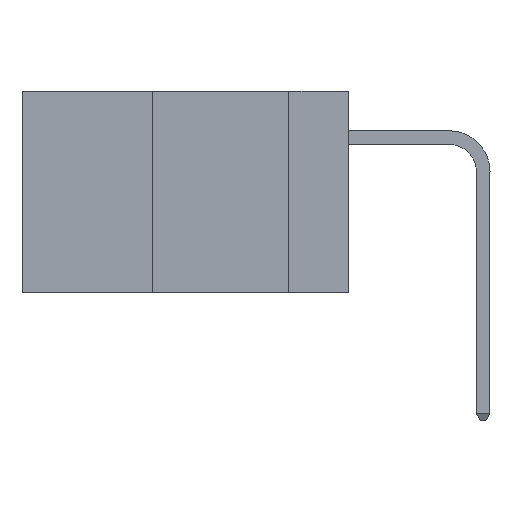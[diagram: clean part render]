
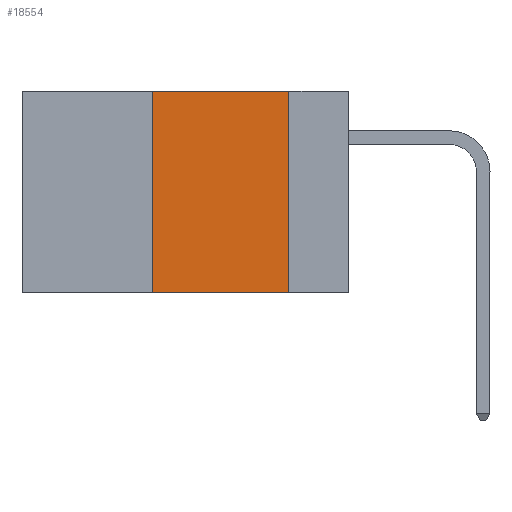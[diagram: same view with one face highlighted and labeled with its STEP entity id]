
A CAD part, left-side view. The second image highlights one B-rep face of the part: STEP entity #18554.
In plain terms, the highlighted planar face has unit normal (-1, 0, 0).
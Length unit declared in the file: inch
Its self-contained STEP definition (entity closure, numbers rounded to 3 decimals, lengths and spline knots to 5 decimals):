
#482 = LINE ( 'NONE', #18165, #28405 ) ;
#672 = EDGE_CURVE ( 'NONE', #12796, #14614, #23000, .T. ) ;
#870 = LINE ( 'NONE', #29139, #24940 ) ;
#1785 = ORIENTED_EDGE ( 'NONE', *, *, #20856, .F. ) ;
#2404 = EDGE_CURVE ( 'NONE', #7783, #14614, #870, .T. ) ;
#2512 = AXIS2_PLACEMENT_3D ( 'NONE', #10956, #13685, #13794 ) ;
#2764 = ORIENTED_EDGE ( 'NONE', *, *, #8146, .F. ) ;
#7552 = FACE_OUTER_BOUND ( 'NONE', #16994, .T. ) ;
#7666 = PLANE ( 'NONE',  #2512 ) ;
#7783 = VERTEX_POINT ( 'NONE', #25748 ) ;
#8146 = EDGE_CURVE ( 'NONE', #18950, #12796, #482, .T. ) ;
#9434 = LINE ( 'NONE', #12547, #24656 ) ;
#10307 = DIRECTION ( 'NONE',  ( 0., -1., 0. ) ) ;
#10956 = CARTESIAN_POINT ( 'NONE',  ( 0., 0.6, 0. ) ) ;
#12547 = CARTESIAN_POINT ( 'NONE',  ( 0., 0.36, 0. ) ) ;
#12796 = VERTEX_POINT ( 'NONE', #34875 ) ;
#13685 = DIRECTION ( 'NONE',  ( 1., 0., 0. ) ) ;
#13794 = DIRECTION ( 'NONE',  ( 0., 0., -1. ) ) ;
#14208 = CARTESIAN_POINT ( 'NONE',  ( 0., 0.11, 0. ) ) ;
#14614 = VERTEX_POINT ( 'NONE', #25064 ) ;
#16994 = EDGE_LOOP ( 'NONE', ( #18665, #2764, #1785, #18248 ) ) ;
#18059 = DIRECTION ( 'NONE',  ( 0., -1., 0. ) ) ;
#18165 = CARTESIAN_POINT ( 'NONE',  ( 0., 0.6, 0. ) ) ;
#18248 = ORIENTED_EDGE ( 'NONE', *, *, #2404, .T. ) ;
#18554 = ADVANCED_FACE ( 'NONE', ( #7552 ), #7666, .F. ) ;
#18665 = ORIENTED_EDGE ( 'NONE', *, *, #672, .F. ) ;
#18950 = VERTEX_POINT ( 'NONE', #26186 ) ;
#20592 = DIRECTION ( 'NONE',  ( 0., 0., 1. ) ) ;
#20856 = EDGE_CURVE ( 'NONE', #7783, #18950, #9434, .T. ) ;
#23000 = LINE ( 'NONE', #14208, #34374 ) ;
#24656 = VECTOR ( 'NONE', #20592, 39.37008 ) ;
#24940 = VECTOR ( 'NONE', #10307, 39.37008 ) ;
#25064 = CARTESIAN_POINT ( 'NONE',  ( 0., 0.11, -0.37 ) ) ;
#25748 = CARTESIAN_POINT ( 'NONE',  ( 0., 0.36, -0.37 ) ) ;
#26186 = CARTESIAN_POINT ( 'NONE',  ( 0., 0.36, 0. ) ) ;
#28060 = DIRECTION ( 'NONE',  ( 0., 0., -1. ) ) ;
#28405 = VECTOR ( 'NONE', #18059, 39.37008 ) ;
#29139 = CARTESIAN_POINT ( 'NONE',  ( 0., 0.6, -0.37 ) ) ;
#34374 = VECTOR ( 'NONE', #28060, 39.37008 ) ;
#34875 = CARTESIAN_POINT ( 'NONE',  ( 0., 0.11, 0. ) ) ;
